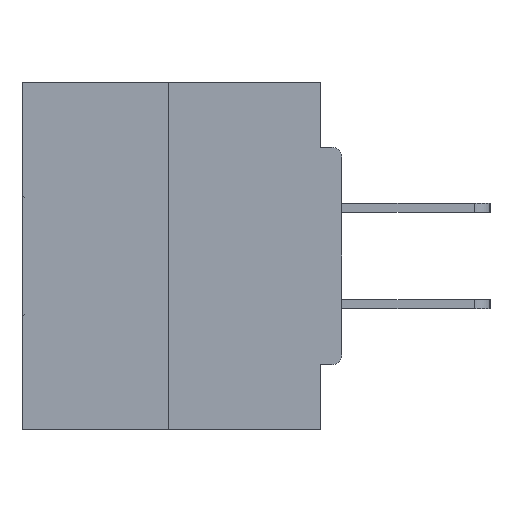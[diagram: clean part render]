
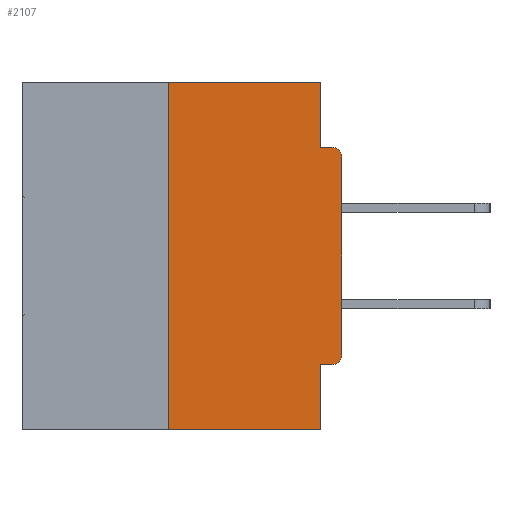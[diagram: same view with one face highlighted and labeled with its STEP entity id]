
A CAD part, left-side view. The second image highlights one B-rep face of the part: STEP entity #2107.
In plain terms, the highlighted planar face has unit normal (-1, 0, 0).
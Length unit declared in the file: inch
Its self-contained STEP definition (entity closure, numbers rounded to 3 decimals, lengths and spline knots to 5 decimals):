
#611 = CARTESIAN_POINT ( 'NONE',  ( 0., 0., -0.1085 ) ) ;
#739 = LINE ( 'NONE', #23983, #27030 ) ;
#1189 = CARTESIAN_POINT ( 'NONE',  ( 0., 0.031, -0.5 ) ) ;
#1693 = CARTESIAN_POINT ( 'NONE',  ( 0., 0.015, -0.3915 ) ) ;
#1904 = CARTESIAN_POINT ( 'NONE',  ( 0., 0., -0.0935 ) ) ;
#1952 = VERTEX_POINT ( 'NONE', #11196 ) ;
#2107 = ADVANCED_FACE ( 'NONE', ( #9749 ), #7041, .F. ) ;
#2478 = LINE ( 'NONE', #17283, #20691 ) ;
#2544 = DIRECTION ( 'NONE',  ( 0., -1., 0. ) ) ;
#2663 = LINE ( 'NONE', #1904, #39666 ) ;
#3757 = DIRECTION ( 'NONE',  ( 0., -1., 0. ) ) ;
#4411 = ORIENTED_EDGE ( 'NONE', *, *, #14695, .F. ) ;
#4953 = CARTESIAN_POINT ( 'NONE',  ( 0., 0.25, 0. ) ) ;
#5349 = CARTESIAN_POINT ( 'NONE',  ( 0., 0.031, -0.0935 ) ) ;
#5409 = VECTOR ( 'NONE', #2544, 39.37008 ) ;
#6584 = LINE ( 'NONE', #19924, #7072 ) ;
#7041 = PLANE ( 'NONE',  #31655 ) ;
#7072 = VECTOR ( 'NONE', #17111, 39.37008 ) ;
#7788 = CARTESIAN_POINT ( 'NONE',  ( 0., 0., -0.3915 ) ) ;
#7998 = DIRECTION ( 'NONE',  ( 0., 0., 1. ) ) ;
#8341 = DIRECTION ( 'NONE',  ( -1., 0., 0. ) ) ;
#9417 = ORIENTED_EDGE ( 'NONE', *, *, #10054, .F. ) ;
#9749 = FACE_OUTER_BOUND ( 'NONE', #35325, .T. ) ;
#9854 = VERTEX_POINT ( 'NONE', #17241 ) ;
#9866 = CARTESIAN_POINT ( 'NONE',  ( 0., 0.015, -0.1085 ) ) ;
#10054 = EDGE_CURVE ( 'NONE', #30521, #39353, #34257, .T. ) ;
#10712 = ORIENTED_EDGE ( 'NONE', *, *, #11925, .F. ) ;
#11165 = VECTOR ( 'NONE', #3757, 39.37008 ) ;
#11196 = CARTESIAN_POINT ( 'NONE',  ( 0., 0.25, -0.5 ) ) ;
#11925 = EDGE_CURVE ( 'NONE', #1952, #30521, #739, .T. ) ;
#12078 = VECTOR ( 'NONE', #12360, 39.37008 ) ;
#12360 = DIRECTION ( 'NONE',  ( 0., 0., -1. ) ) ;
#12470 = AXIS2_PLACEMENT_3D ( 'NONE', #9866, #19665, #16540 ) ;
#14575 = ORIENTED_EDGE ( 'NONE', *, *, #31103, .F. ) ;
#14695 = EDGE_CURVE ( 'NONE', #15710, #9854, #35040, .T. ) ;
#15245 = ORIENTED_EDGE ( 'NONE', *, *, #15748, .F. ) ;
#15302 = CARTESIAN_POINT ( 'NONE',  ( 0., 0.015, -0.4065 ) ) ;
#15710 = VERTEX_POINT ( 'NONE', #15302 ) ;
#15748 = EDGE_CURVE ( 'NONE', #39353, #16588, #6584, .T. ) ;
#15827 = CARTESIAN_POINT ( 'NONE',  ( 0., 0.46, 0. ) ) ;
#16161 = EDGE_CURVE ( 'NONE', #1952, #20374, #32417, .T. ) ;
#16400 = CARTESIAN_POINT ( 'NONE',  ( 0., 0.46, 0. ) ) ;
#16540 = DIRECTION ( 'NONE',  ( 0., 0., -1. ) ) ;
#16588 = VERTEX_POINT ( 'NONE', #5349 ) ;
#16710 = VERTEX_POINT ( 'NONE', #28203 ) ;
#17111 = DIRECTION ( 'NONE',  ( 0., 0., -1. ) ) ;
#17241 = CARTESIAN_POINT ( 'NONE',  ( 0., 0.031, -0.4065 ) ) ;
#17283 = CARTESIAN_POINT ( 'NONE',  ( 0., 0., 0. ) ) ;
#18756 = ORIENTED_EDGE ( 'NONE', *, *, #38183, .T. ) ;
#19665 = DIRECTION ( 'NONE',  ( -1., 0., 0. ) ) ;
#19924 = CARTESIAN_POINT ( 'NONE',  ( 0., 0.031, 0. ) ) ;
#20020 = ORIENTED_EDGE ( 'NONE', *, *, #16161, .T. ) ;
#20374 = VERTEX_POINT ( 'NONE', #1189 ) ;
#20691 = VECTOR ( 'NONE', #23605, 39.37008 ) ;
#20860 = VERTEX_POINT ( 'NONE', #7788 ) ;
#22865 = DIRECTION ( 'NONE',  ( 1., 0., 0. ) ) ;
#23201 = EDGE_CURVE ( 'NONE', #34698, #16710, #41638, .T. ) ;
#23605 = DIRECTION ( 'NONE',  ( 0., 0., 1. ) ) ;
#23651 = CARTESIAN_POINT ( 'NONE',  ( 0., 0.031, 0. ) ) ;
#23983 = CARTESIAN_POINT ( 'NONE',  ( 0., 0.25, 0. ) ) ;
#26128 = DIRECTION ( 'NONE',  ( 0., 0., -1. ) ) ;
#26886 = DIRECTION ( 'NONE',  ( 0., 1., 0. ) ) ;
#27030 = VECTOR ( 'NONE', #7998, 39.37008 ) ;
#28203 = CARTESIAN_POINT ( 'NONE',  ( 0., 0.015, -0.0935 ) ) ;
#29218 = LINE ( 'NONE', #31713, #12078 ) ;
#30400 = ORIENTED_EDGE ( 'NONE', *, *, #23201, .T. ) ;
#30521 = VERTEX_POINT ( 'NONE', #4953 ) ;
#30977 = DIRECTION ( 'NONE',  ( 0., 0., -1. ) ) ;
#31103 = EDGE_CURVE ( 'NONE', #9854, #20374, #29218, .T. ) ;
#31655 = AXIS2_PLACEMENT_3D ( 'NONE', #16400, #22865, #26128 ) ;
#31713 = CARTESIAN_POINT ( 'NONE',  ( 0., 0.031, -0.5 ) ) ;
#32336 = CARTESIAN_POINT ( 'NONE',  ( 0., 0.46, -0.5 ) ) ;
#32417 = LINE ( 'NONE', #32336, #11165 ) ;
#33215 = EDGE_CURVE ( 'NONE', #15710, #20860, #35550, .T. ) ;
#33282 = CARTESIAN_POINT ( 'NONE',  ( 0., 0., -0.4065 ) ) ;
#33337 = EDGE_CURVE ( 'NONE', #16588, #16710, #2663, .T. ) ;
#34257 = LINE ( 'NONE', #15827, #5409 ) ;
#34579 = VECTOR ( 'NONE', #26886, 39.37008 ) ;
#34698 = VERTEX_POINT ( 'NONE', #611 ) ;
#35040 = LINE ( 'NONE', #33282, #34579 ) ;
#35325 = EDGE_LOOP ( 'NONE', ( #9417, #10712, #20020, #14575, #4411, #39475, #18756, #30400, #36224, #15245 ) ) ;
#35550 = CIRCLE ( 'NONE', #41172, 0.015 ) ;
#36224 = ORIENTED_EDGE ( 'NONE', *, *, #33337, .F. ) ;
#38183 = EDGE_CURVE ( 'NONE', #20860, #34698, #2478, .T. ) ;
#39353 = VERTEX_POINT ( 'NONE', #23651 ) ;
#39475 = ORIENTED_EDGE ( 'NONE', *, *, #33215, .T. ) ;
#39569 = DIRECTION ( 'NONE',  ( 0., -1., 0. ) ) ;
#39666 = VECTOR ( 'NONE', #39569, 39.37008 ) ;
#41172 = AXIS2_PLACEMENT_3D ( 'NONE', #1693, #8341, #30977 ) ;
#41638 = CIRCLE ( 'NONE', #12470, 0.015 ) ;
